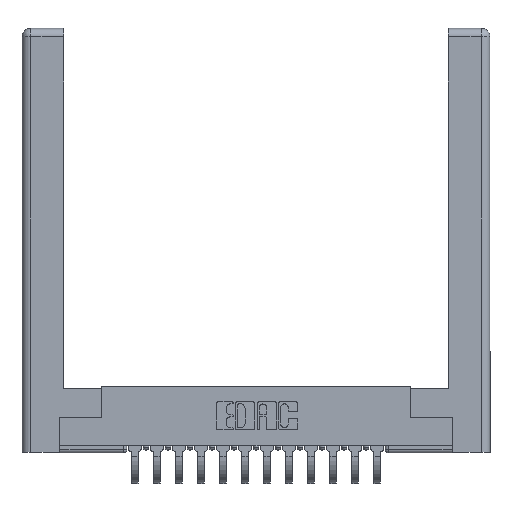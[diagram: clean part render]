
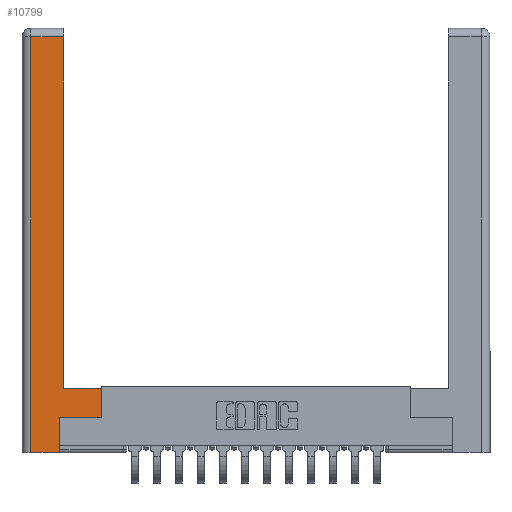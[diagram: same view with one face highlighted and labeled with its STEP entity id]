
A CAD part, top view. The second image highlights one B-rep face of the part: STEP entity #10799.
In plain terms, the highlighted planar face has unit normal (0, 0, 1).
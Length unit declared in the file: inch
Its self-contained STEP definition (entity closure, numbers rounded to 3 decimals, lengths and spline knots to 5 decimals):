
#483 = DIRECTION ( 'NONE',  ( -1., 0., 0. ) ) ;
#746 = LINE ( 'NONE', #12529, #17186 ) ;
#821 = DIRECTION ( 'NONE',  ( 0., 1., 0. ) ) ;
#1308 = VERTEX_POINT ( 'NONE', #14997 ) ;
#1761 = LINE ( 'NONE', #6240, #15951 ) ;
#1791 = VECTOR ( 'NONE', #2800, 39.37008 ) ;
#1903 = VECTOR ( 'NONE', #821, 39.37008 ) ;
#1995 = VERTEX_POINT ( 'NONE', #5684 ) ;
#2296 = LINE ( 'NONE', #9117, #1903 ) ;
#2716 = CARTESIAN_POINT ( 'NONE',  ( 0.295, 0.45, 0. ) ) ;
#2800 = DIRECTION ( 'NONE',  ( -1., 0., 0. ) ) ;
#3310 = ORIENTED_EDGE ( 'NONE', *, *, #17335, .T. ) ;
#3836 = LINE ( 'NONE', #18150, #9650 ) ;
#4825 = AXIS2_PLACEMENT_3D ( 'NONE', #7474, #14478, #17385 ) ;
#5052 = DIRECTION ( 'NONE',  ( 0., 1., 0. ) ) ;
#5344 = LINE ( 'NONE', #2716, #1791 ) ;
#5420 = ORIENTED_EDGE ( 'NONE', *, *, #17313, .T. ) ;
#5684 = CARTESIAN_POINT ( 'NONE',  ( 0.0615, 2.94, 0. ) ) ;
#6059 = VECTOR ( 'NONE', #483, 39.37008 ) ;
#6173 = LINE ( 'NONE', #7577, #6059 ) ;
#6240 = CARTESIAN_POINT ( 'NONE',  ( 0.565, 0.45, 0. ) ) ;
#7080 = EDGE_CURVE ( 'NONE', #12375, #1308, #5344, .T. ) ;
#7252 = LINE ( 'NONE', #8838, #11225 ) ;
#7474 = CARTESIAN_POINT ( 'NONE',  ( 0., 0., 0. ) ) ;
#7577 = CARTESIAN_POINT ( 'NONE',  ( 0.0615, 2.94, 0. ) ) ;
#7692 = ORIENTED_EDGE ( 'NONE', *, *, #10159, .T. ) ;
#7734 = ORIENTED_EDGE ( 'NONE', *, *, #8248, .T. ) ;
#7858 = EDGE_LOOP ( 'NONE', ( #15771, #5420, #15686, #7734, #3310, #7692, #17644, #14607 ) ) ;
#8248 = EDGE_CURVE ( 'NONE', #8685, #10235, #7252, .T. ) ;
#8414 = CARTESIAN_POINT ( 'NONE',  ( 0.265, 0.245, 0. ) ) ;
#8436 = VERTEX_POINT ( 'NONE', #12860 ) ;
#8442 = CARTESIAN_POINT ( 'NONE',  ( 0.265, 0., 0. ) ) ;
#8685 = VERTEX_POINT ( 'NONE', #17163 ) ;
#8838 = CARTESIAN_POINT ( 'NONE',  ( 0.265, 0., 0. ) ) ;
#9117 = CARTESIAN_POINT ( 'NONE',  ( 0.295, 3., 0. ) ) ;
#9206 = EDGE_CURVE ( 'NONE', #1995, #8685, #746, .T. ) ;
#9470 = CARTESIAN_POINT ( 'NONE',  ( 0.565, 0.245, 0. ) ) ;
#9521 = DIRECTION ( 'NONE',  ( 0., -1., 0. ) ) ;
#9650 = VECTOR ( 'NONE', #5052, 39.37008 ) ;
#10007 = PLANE ( 'NONE',  #4825 ) ;
#10159 = EDGE_CURVE ( 'NONE', #14458, #12751, #14817, .T. ) ;
#10191 = FACE_OUTER_BOUND ( 'NONE', #7858, .T. ) ;
#10235 = VERTEX_POINT ( 'NONE', #8442 ) ;
#10799 = ADVANCED_FACE ( 'NONE', ( #10191 ), #10007, .F. ) ;
#11225 = VECTOR ( 'NONE', #17641, 39.37008 ) ;
#12375 = VERTEX_POINT ( 'NONE', #17072 ) ;
#12529 = CARTESIAN_POINT ( 'NONE',  ( 0.0615, 0., 0. ) ) ;
#12751 = VERTEX_POINT ( 'NONE', #9470 ) ;
#12847 = DIRECTION ( 'NONE',  ( 1., 0., 0. ) ) ;
#12860 = CARTESIAN_POINT ( 'NONE',  ( 0.295, 2.94, 0. ) ) ;
#13776 = VECTOR ( 'NONE', #12847, 39.37008 ) ;
#13876 = CARTESIAN_POINT ( 'NONE',  ( 0.565, 0.245, 0. ) ) ;
#14458 = VERTEX_POINT ( 'NONE', #8414 ) ;
#14478 = DIRECTION ( 'NONE',  ( 0., 0., -1. ) ) ;
#14607 = ORIENTED_EDGE ( 'NONE', *, *, #7080, .T. ) ;
#14817 = LINE ( 'NONE', #13876, #13776 ) ;
#14997 = CARTESIAN_POINT ( 'NONE',  ( 0.295, 0.45, 0. ) ) ;
#15686 = ORIENTED_EDGE ( 'NONE', *, *, #9206, .T. ) ;
#15771 = ORIENTED_EDGE ( 'NONE', *, *, #18305, .T. ) ;
#15951 = VECTOR ( 'NONE', #15985, 39.37008 ) ;
#15985 = DIRECTION ( 'NONE',  ( 0., 1., 0. ) ) ;
#17072 = CARTESIAN_POINT ( 'NONE',  ( 0.565, 0.45, 0. ) ) ;
#17163 = CARTESIAN_POINT ( 'NONE',  ( 0.0615, 0., 0. ) ) ;
#17186 = VECTOR ( 'NONE', #9521, 39.37008 ) ;
#17313 = EDGE_CURVE ( 'NONE', #8436, #1995, #6173, .T. ) ;
#17335 = EDGE_CURVE ( 'NONE', #10235, #14458, #3836, .T. ) ;
#17385 = DIRECTION ( 'NONE',  ( -1., 0., 0. ) ) ;
#17641 = DIRECTION ( 'NONE',  ( 1., 0., 0. ) ) ;
#17644 = ORIENTED_EDGE ( 'NONE', *, *, #17750, .T. ) ;
#17750 = EDGE_CURVE ( 'NONE', #12751, #12375, #1761, .T. ) ;
#18150 = CARTESIAN_POINT ( 'NONE',  ( 0.265, 0.245, 0. ) ) ;
#18305 = EDGE_CURVE ( 'NONE', #1308, #8436, #2296, .T. ) ;
